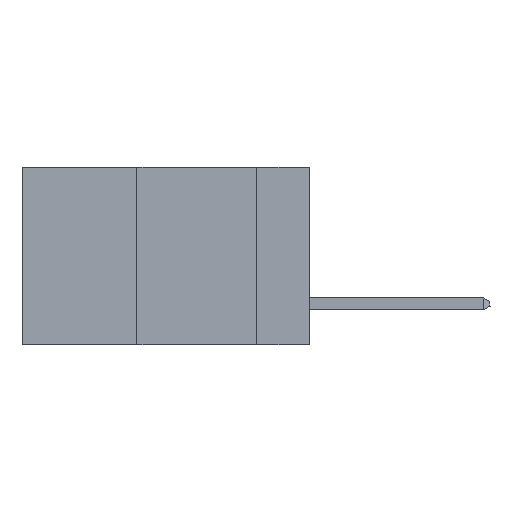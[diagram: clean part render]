
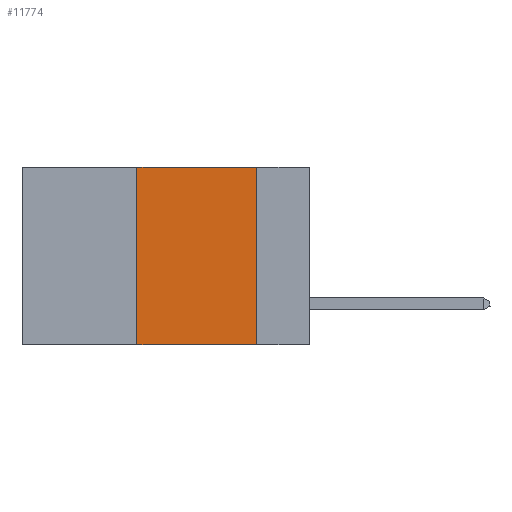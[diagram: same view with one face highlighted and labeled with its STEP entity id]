
A CAD part, left-side view. The second image highlights one B-rep face of the part: STEP entity #11774.
In plain terms, the highlighted planar face has unit normal (-1, 0, 0).
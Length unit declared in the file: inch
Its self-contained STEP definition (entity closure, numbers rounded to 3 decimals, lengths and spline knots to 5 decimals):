
#278 = DIRECTION ( 'NONE',  ( 1., 0., 0. ) ) ;
#738 = VERTEX_POINT ( 'NONE', #27316 ) ;
#1070 = ORIENTED_EDGE ( 'NONE', *, *, #27838, .T. ) ;
#1080 = EDGE_CURVE ( 'NONE', #16089, #14424, #2426, .T. ) ;
#1927 = LINE ( 'NONE', #10680, #15710 ) ;
#2426 = LINE ( 'NONE', #2476, #11984 ) ;
#2476 = CARTESIAN_POINT ( 'NONE',  ( 0., 0.36, 0. ) ) ;
#2840 = ORIENTED_EDGE ( 'NONE', *, *, #1080, .F. ) ;
#3749 = DIRECTION ( 'NONE',  ( 0., 0., -1. ) ) ;
#3872 = CARTESIAN_POINT ( 'NONE',  ( 0., 0.11, 0. ) ) ;
#4884 = LINE ( 'NONE', #7218, #14407 ) ;
#6031 = DIRECTION ( 'NONE',  ( 0., -1., 0. ) ) ;
#6920 = AXIS2_PLACEMENT_3D ( 'NONE', #26440, #278, #3749 ) ;
#7218 = CARTESIAN_POINT ( 'NONE',  ( 0., 0.6, -0.37 ) ) ;
#7608 = ORIENTED_EDGE ( 'NONE', *, *, #12979, .F. ) ;
#8503 = VECTOR ( 'NONE', #22105, 39.37008 ) ;
#10680 = CARTESIAN_POINT ( 'NONE',  ( 0., 0.6, 0. ) ) ;
#11774 = ADVANCED_FACE ( 'NONE', ( #12429 ), #15440, .F. ) ;
#11984 = VECTOR ( 'NONE', #26217, 39.37008 ) ;
#12429 = FACE_OUTER_BOUND ( 'NONE', #26922, .T. ) ;
#12441 = ORIENTED_EDGE ( 'NONE', *, *, #29255, .F. ) ;
#12979 = EDGE_CURVE ( 'NONE', #738, #23824, #26939, .T. ) ;
#14407 = VECTOR ( 'NONE', #20901, 39.37008 ) ;
#14424 = VERTEX_POINT ( 'NONE', #27276 ) ;
#15440 = PLANE ( 'NONE',  #6920 ) ;
#15710 = VECTOR ( 'NONE', #6031, 39.37008 ) ;
#16089 = VERTEX_POINT ( 'NONE', #22318 ) ;
#16548 = CARTESIAN_POINT ( 'NONE',  ( 0., 0.11, -0.37 ) ) ;
#20901 = DIRECTION ( 'NONE',  ( 0., -1., 0. ) ) ;
#22105 = DIRECTION ( 'NONE',  ( 0., 0., -1. ) ) ;
#22318 = CARTESIAN_POINT ( 'NONE',  ( 0., 0.36, -0.37 ) ) ;
#23824 = VERTEX_POINT ( 'NONE', #16548 ) ;
#26217 = DIRECTION ( 'NONE',  ( 0., 0., 1. ) ) ;
#26440 = CARTESIAN_POINT ( 'NONE',  ( 0., 0.6, 0. ) ) ;
#26922 = EDGE_LOOP ( 'NONE', ( #7608, #12441, #2840, #1070 ) ) ;
#26939 = LINE ( 'NONE', #3872, #8503 ) ;
#27276 = CARTESIAN_POINT ( 'NONE',  ( 0., 0.36, 0. ) ) ;
#27316 = CARTESIAN_POINT ( 'NONE',  ( 0., 0.11, 0. ) ) ;
#27838 = EDGE_CURVE ( 'NONE', #16089, #23824, #4884, .T. ) ;
#29255 = EDGE_CURVE ( 'NONE', #14424, #738, #1927, .T. ) ;
